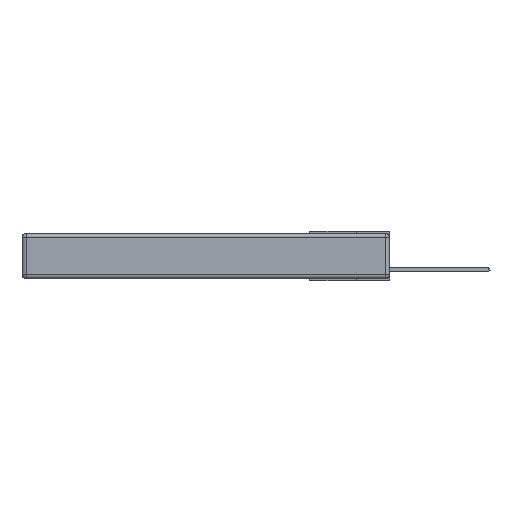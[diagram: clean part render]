
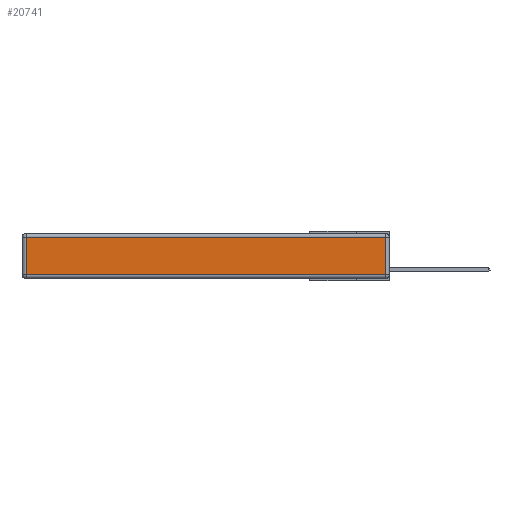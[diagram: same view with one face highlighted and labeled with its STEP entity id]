
A CAD part, left-side view. The second image highlights one B-rep face of the part: STEP entity #20741.
In plain terms, the highlighted planar face has unit normal (-1, 0, 0).
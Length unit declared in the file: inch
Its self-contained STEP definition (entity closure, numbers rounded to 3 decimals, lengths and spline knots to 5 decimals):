
#182 = LINE ( 'NONE', #19350, #8934 ) ;
#586 = DIRECTION ( 'NONE',  ( 0., 1., 0. ) ) ;
#873 = VERTEX_POINT ( 'NONE', #14884 ) ;
#2323 = EDGE_CURVE ( 'NONE', #10072, #873, #182, .T. ) ;
#2351 = DIRECTION ( 'NONE',  ( -1., 0., 0. ) ) ;
#2826 = ORIENTED_EDGE ( 'NONE', *, *, #2323, .T. ) ;
#4320 = DIRECTION ( 'NONE',  ( 0., 0., 1. ) ) ;
#5310 = DIRECTION ( 'NONE',  ( 0., 0., 1. ) ) ;
#6123 = LINE ( 'NONE', #19972, #7152 ) ;
#6757 = VECTOR ( 'NONE', #5310, 39.37008 ) ;
#7152 = VECTOR ( 'NONE', #13785, 39.37008 ) ;
#7231 = DIRECTION ( 'NONE',  ( 0., 0., -1. ) ) ;
#7403 = ORIENTED_EDGE ( 'NONE', *, *, #22919, .T. ) ;
#8064 = LINE ( 'NONE', #20005, #6757 ) ;
#8934 = VECTOR ( 'NONE', #586, 39.37008 ) ;
#10072 = VERTEX_POINT ( 'NONE', #27056 ) ;
#11021 = ORIENTED_EDGE ( 'NONE', *, *, #20357, .T. ) ;
#11859 = FACE_OUTER_BOUND ( 'NONE', #23535, .T. ) ;
#12745 = ORIENTED_EDGE ( 'NONE', *, *, #27333, .T. ) ;
#13031 = PLANE ( 'NONE',  #19855 ) ;
#13785 = DIRECTION ( 'NONE',  ( 0., -1., 0. ) ) ;
#14396 = CARTESIAN_POINT ( 'NONE',  ( 0., 0.03, -0.313 ) ) ;
#14884 = CARTESIAN_POINT ( 'NONE',  ( 0., 2.72, -0.03 ) ) ;
#16648 = VERTEX_POINT ( 'NONE', #24745 ) ;
#19350 = CARTESIAN_POINT ( 'NONE',  ( 0., 2.75, -0.03 ) ) ;
#19492 = CARTESIAN_POINT ( 'NONE',  ( 0., 0., -0.343 ) ) ;
#19855 = AXIS2_PLACEMENT_3D ( 'NONE', #19492, #2351, #4320 ) ;
#19972 = CARTESIAN_POINT ( 'NONE',  ( 0., 0., -0.313 ) ) ;
#20005 = CARTESIAN_POINT ( 'NONE',  ( 0., 0.03, -0.343 ) ) ;
#20068 = CARTESIAN_POINT ( 'NONE',  ( 0., 2.72, -0.343 ) ) ;
#20357 = EDGE_CURVE ( 'NONE', #873, #16648, #20566, .T. ) ;
#20566 = LINE ( 'NONE', #20068, #27515 ) ;
#20741 = ADVANCED_FACE ( 'NONE', ( #11859 ), #13031, .T. ) ;
#22919 = EDGE_CURVE ( 'NONE', #26467, #10072, #8064, .T. ) ;
#23535 = EDGE_LOOP ( 'NONE', ( #12745, #7403, #2826, #11021 ) ) ;
#24745 = CARTESIAN_POINT ( 'NONE',  ( 0., 2.72, -0.313 ) ) ;
#26467 = VERTEX_POINT ( 'NONE', #14396 ) ;
#27056 = CARTESIAN_POINT ( 'NONE',  ( 0., 0.03, -0.03 ) ) ;
#27333 = EDGE_CURVE ( 'NONE', #16648, #26467, #6123, .T. ) ;
#27515 = VECTOR ( 'NONE', #7231, 39.37008 ) ;
